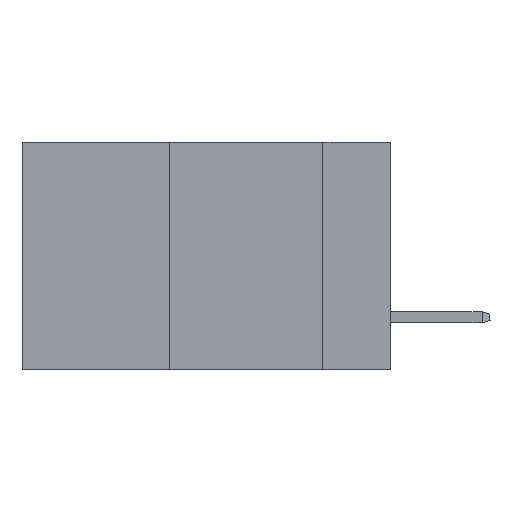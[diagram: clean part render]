
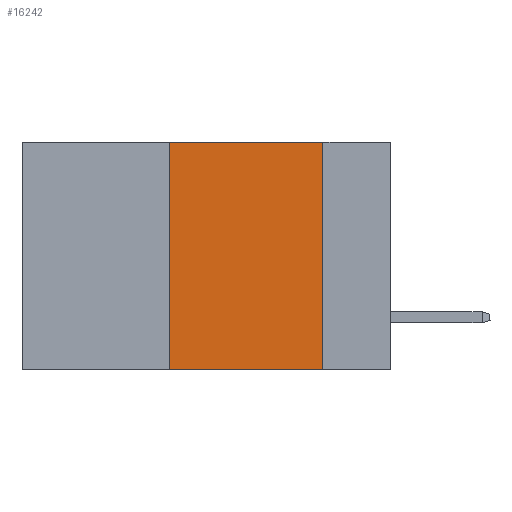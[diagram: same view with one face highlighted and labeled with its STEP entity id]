
A CAD part, left-side view. The second image highlights one B-rep face of the part: STEP entity #16242.
In plain terms, the highlighted planar face has unit normal (-1, 0, 0).
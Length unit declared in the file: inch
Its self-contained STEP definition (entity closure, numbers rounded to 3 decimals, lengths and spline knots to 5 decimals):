
#1060 = VECTOR ( 'NONE', #21121, 39.37008 ) ;
#1363 = ORIENTED_EDGE ( 'NONE', *, *, #26046, .F. ) ;
#3346 = CARTESIAN_POINT ( 'NONE',  ( 0., 0.6, -0.37 ) ) ;
#3885 = ORIENTED_EDGE ( 'NONE', *, *, #13525, .F. ) ;
#5681 = DIRECTION ( 'NONE',  ( 0., 0., -1. ) ) ;
#7933 = CARTESIAN_POINT ( 'NONE',  ( 0., 0.36, 0. ) ) ;
#10295 = DIRECTION ( 'NONE',  ( 0., -1., 0. ) ) ;
#10590 = DIRECTION ( 'NONE',  ( 1., 0., 0. ) ) ;
#12471 = CARTESIAN_POINT ( 'NONE',  ( 0., 0.11, 0. ) ) ;
#13237 = LINE ( 'NONE', #3346, #23623 ) ;
#13253 = VERTEX_POINT ( 'NONE', #22244 ) ;
#13502 = VECTOR ( 'NONE', #5681, 39.37008 ) ;
#13525 = EDGE_CURVE ( 'NONE', #15102, #13253, #17000, .T. ) ;
#15102 = VERTEX_POINT ( 'NONE', #32776 ) ;
#15506 = PLANE ( 'NONE',  #22120 ) ;
#15935 = ORIENTED_EDGE ( 'NONE', *, *, #27257, .F. ) ;
#16242 = ADVANCED_FACE ( 'NONE', ( #28364 ), #15506, .F. ) ;
#17000 = LINE ( 'NONE', #7933, #1060 ) ;
#18285 = CARTESIAN_POINT ( 'NONE',  ( 0., 0.6, 0. ) ) ;
#18434 = CARTESIAN_POINT ( 'NONE',  ( 0., 0.6, 0. ) ) ;
#19585 = VECTOR ( 'NONE', #10295, 39.37008 ) ;
#20651 = DIRECTION ( 'NONE',  ( 0., 0., -1. ) ) ;
#20729 = EDGE_LOOP ( 'NONE', ( #15935, #1363, #3885, #26947 ) ) ;
#20954 = CARTESIAN_POINT ( 'NONE',  ( 0., 0.11, 0. ) ) ;
#21121 = DIRECTION ( 'NONE',  ( 0., 0., 1. ) ) ;
#22120 = AXIS2_PLACEMENT_3D ( 'NONE', #18285, #10590, #20651 ) ;
#22244 = CARTESIAN_POINT ( 'NONE',  ( 0., 0.36, 0. ) ) ;
#22370 = LINE ( 'NONE', #18434, #19585 ) ;
#23623 = VECTOR ( 'NONE', #32214, 39.37008 ) ;
#24259 = LINE ( 'NONE', #20954, #13502 ) ;
#25165 = EDGE_CURVE ( 'NONE', #15102, #26836, #13237, .T. ) ;
#26046 = EDGE_CURVE ( 'NONE', #13253, #27038, #22370, .T. ) ;
#26836 = VERTEX_POINT ( 'NONE', #27214 ) ;
#26947 = ORIENTED_EDGE ( 'NONE', *, *, #25165, .T. ) ;
#27038 = VERTEX_POINT ( 'NONE', #12471 ) ;
#27214 = CARTESIAN_POINT ( 'NONE',  ( 0., 0.11, -0.37 ) ) ;
#27257 = EDGE_CURVE ( 'NONE', #27038, #26836, #24259, .T. ) ;
#28364 = FACE_OUTER_BOUND ( 'NONE', #20729, .T. ) ;
#32214 = DIRECTION ( 'NONE',  ( 0., -1., 0. ) ) ;
#32776 = CARTESIAN_POINT ( 'NONE',  ( 0., 0.36, -0.37 ) ) ;
